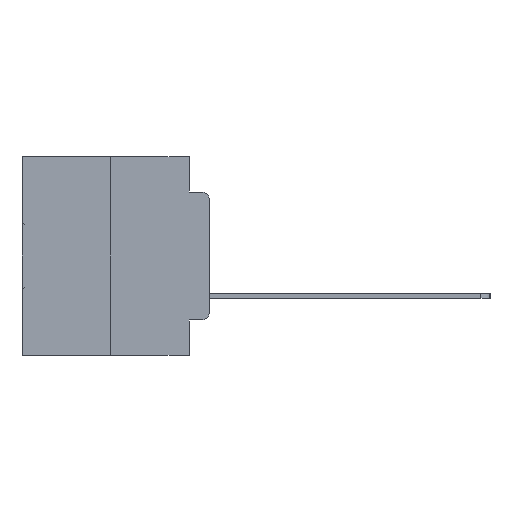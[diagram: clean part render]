
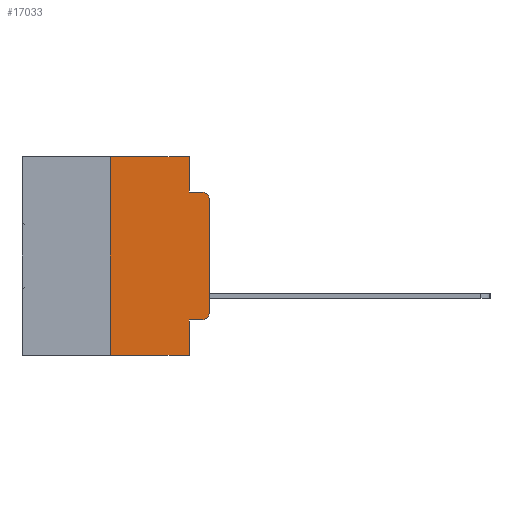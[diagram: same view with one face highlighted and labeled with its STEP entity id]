
A CAD part, left-side view. The second image highlights one B-rep face of the part: STEP entity #17033.
In plain terms, the highlighted planar face has unit normal (-1, 0, 0).
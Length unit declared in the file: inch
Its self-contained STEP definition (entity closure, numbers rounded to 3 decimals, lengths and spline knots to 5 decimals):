
#252 = VERTEX_POINT ( 'NONE', #14850 ) ;
#990 = ORIENTED_EDGE ( 'NONE', *, *, #18573, .F. ) ;
#1115 = CARTESIAN_POINT ( 'NONE',  ( 0., 0.051, -0.0885 ) ) ;
#2175 = DIRECTION ( 'NONE',  ( 0., 0., 1. ) ) ;
#2446 = CARTESIAN_POINT ( 'NONE',  ( 0., 0.051, -0.0885 ) ) ;
#2524 = EDGE_CURVE ( 'NONE', #5758, #2970, #29558, .T. ) ;
#2970 = VERTEX_POINT ( 'NONE', #21979 ) ;
#3395 = ORIENTED_EDGE ( 'NONE', *, *, #17707, .T. ) ;
#5014 = CARTESIAN_POINT ( 'NONE',  ( 0., 0., -0.3915 ) ) ;
#5758 = VERTEX_POINT ( 'NONE', #5014 ) ;
#6144 = VECTOR ( 'NONE', #26888, 39.37008 ) ;
#6301 = CARTESIAN_POINT ( 'NONE',  ( 0., 0.02, -0.3915 ) ) ;
#6865 = ORIENTED_EDGE ( 'NONE', *, *, #22672, .F. ) ;
#6908 = CARTESIAN_POINT ( 'NONE',  ( 0., 0.051, -0.4115 ) ) ;
#7095 = VECTOR ( 'NONE', #25287, 39.37008 ) ;
#7397 = CARTESIAN_POINT ( 'NONE',  ( 0., 0.051, 0. ) ) ;
#7798 = VECTOR ( 'NONE', #22179, 39.37008 ) ;
#8592 = ORIENTED_EDGE ( 'NONE', *, *, #26664, .T. ) ;
#8744 = VECTOR ( 'NONE', #21760, 39.37008 ) ;
#8849 = DIRECTION ( 'NONE',  ( -1., 0., 0. ) ) ;
#8956 = DIRECTION ( 'NONE',  ( 0., 0., -1. ) ) ;
#9239 = VECTOR ( 'NONE', #2175, 39.37008 ) ;
#9633 = CARTESIAN_POINT ( 'NONE',  ( 0., 0.02, -0.0885 ) ) ;
#9834 = VERTEX_POINT ( 'NONE', #2446 ) ;
#10492 = EDGE_LOOP ( 'NONE', ( #15350, #18799, #27840, #26714, #18135, #6865, #13405, #990, #8592, #3395 ) ) ;
#10889 = VERTEX_POINT ( 'NONE', #11361 ) ;
#11210 = CIRCLE ( 'NONE', #26092, 0.02 ) ;
#11361 = CARTESIAN_POINT ( 'NONE',  ( 0., 0.051, -0.5 ) ) ;
#11922 = VERTEX_POINT ( 'NONE', #32232 ) ;
#12493 = DIRECTION ( 'NONE',  ( 0., 0., -1. ) ) ;
#12929 = CARTESIAN_POINT ( 'NONE',  ( 0., 0.25, 0. ) ) ;
#13405 = ORIENTED_EDGE ( 'NONE', *, *, #26143, .T. ) ;
#14701 = LINE ( 'NONE', #6908, #7798 ) ;
#14850 = CARTESIAN_POINT ( 'NONE',  ( 0., 0.051, -0.4115 ) ) ;
#14866 = LINE ( 'NONE', #20136, #27559 ) ;
#14972 = CARTESIAN_POINT ( 'NONE',  ( 0., 0.473, 0. ) ) ;
#15350 = ORIENTED_EDGE ( 'NONE', *, *, #2524, .T. ) ;
#15616 = LINE ( 'NONE', #7397, #7095 ) ;
#16133 = FACE_OUTER_BOUND ( 'NONE', #10492, .T. ) ;
#16263 = EDGE_CURVE ( 'NONE', #32279, #20979, #26595, .T. ) ;
#16665 = LINE ( 'NONE', #26511, #22610 ) ;
#17033 = ADVANCED_FACE ( 'NONE', ( #16133 ), #20043, .F. ) ;
#17178 = LINE ( 'NONE', #1115, #8744 ) ;
#17538 = DIRECTION ( 'NONE',  ( 0., -1., 0. ) ) ;
#17707 = EDGE_CURVE ( 'NONE', #33169, #5758, #27573, .T. ) ;
#17897 = LINE ( 'NONE', #32687, #25439 ) ;
#18135 = ORIENTED_EDGE ( 'NONE', *, *, #16263, .F. ) ;
#18291 = AXIS2_PLACEMENT_3D ( 'NONE', #6301, #24267, #8956 ) ;
#18573 = EDGE_CURVE ( 'NONE', #252, #10889, #15616, .T. ) ;
#18715 = DIRECTION ( 'NONE',  ( 0., 0., -1. ) ) ;
#18799 = ORIENTED_EDGE ( 'NONE', *, *, #32496, .T. ) ;
#20043 = PLANE ( 'NONE',  #31477 ) ;
#20136 = CARTESIAN_POINT ( 'NONE',  ( 0., 0.25, 0. ) ) ;
#20979 = VERTEX_POINT ( 'NONE', #31571 ) ;
#21760 = DIRECTION ( 'NONE',  ( 0., -1., 0. ) ) ;
#21781 = CARTESIAN_POINT ( 'NONE',  ( 0., 0.473, 0. ) ) ;
#21842 = EDGE_CURVE ( 'NONE', #9834, #32703, #17178, .T. ) ;
#21979 = CARTESIAN_POINT ( 'NONE',  ( 0., 0., -0.1085 ) ) ;
#22179 = DIRECTION ( 'NONE',  ( 0., -1., 0. ) ) ;
#22610 = VECTOR ( 'NONE', #18715, 39.37008 ) ;
#22672 = EDGE_CURVE ( 'NONE', #11922, #32279, #14866, .T. ) ;
#22713 = DIRECTION ( 'NONE',  ( 0., 0., 1. ) ) ;
#24161 = CARTESIAN_POINT ( 'NONE',  ( 0., 0.02, -0.1085 ) ) ;
#24267 = DIRECTION ( 'NONE',  ( -1., 0., 0. ) ) ;
#25287 = DIRECTION ( 'NONE',  ( 0., 0., -1. ) ) ;
#25439 = VECTOR ( 'NONE', #17538, 39.37008 ) ;
#26092 = AXIS2_PLACEMENT_3D ( 'NONE', #24161, #8849, #26694 ) ;
#26143 = EDGE_CURVE ( 'NONE', #11922, #10889, #17897, .T. ) ;
#26511 = CARTESIAN_POINT ( 'NONE',  ( 0., 0.051, 0. ) ) ;
#26595 = LINE ( 'NONE', #21781, #6144 ) ;
#26664 = EDGE_CURVE ( 'NONE', #252, #33169, #14701, .T. ) ;
#26694 = DIRECTION ( 'NONE',  ( 0., 0., -1. ) ) ;
#26714 = ORIENTED_EDGE ( 'NONE', *, *, #29267, .F. ) ;
#26888 = DIRECTION ( 'NONE',  ( 0., -1., 0. ) ) ;
#27559 = VECTOR ( 'NONE', #22713, 39.37008 ) ;
#27573 = CIRCLE ( 'NONE', #18291, 0.02 ) ;
#27707 = DIRECTION ( 'NONE',  ( 1., 0., 0. ) ) ;
#27840 = ORIENTED_EDGE ( 'NONE', *, *, #21842, .F. ) ;
#29267 = EDGE_CURVE ( 'NONE', #20979, #9834, #16665, .T. ) ;
#29558 = LINE ( 'NONE', #32379, #9239 ) ;
#31477 = AXIS2_PLACEMENT_3D ( 'NONE', #14972, #27707, #12493 ) ;
#31571 = CARTESIAN_POINT ( 'NONE',  ( 0., 0.051, 0. ) ) ;
#31839 = CARTESIAN_POINT ( 'NONE',  ( 0., 0.02, -0.4115 ) ) ;
#32232 = CARTESIAN_POINT ( 'NONE',  ( 0., 0.25, -0.5 ) ) ;
#32279 = VERTEX_POINT ( 'NONE', #12929 ) ;
#32379 = CARTESIAN_POINT ( 'NONE',  ( 0., 0., 0. ) ) ;
#32496 = EDGE_CURVE ( 'NONE', #2970, #32703, #11210, .T. ) ;
#32687 = CARTESIAN_POINT ( 'NONE',  ( 0., 0.473, -0.5 ) ) ;
#32703 = VERTEX_POINT ( 'NONE', #9633 ) ;
#33169 = VERTEX_POINT ( 'NONE', #31839 ) ;
